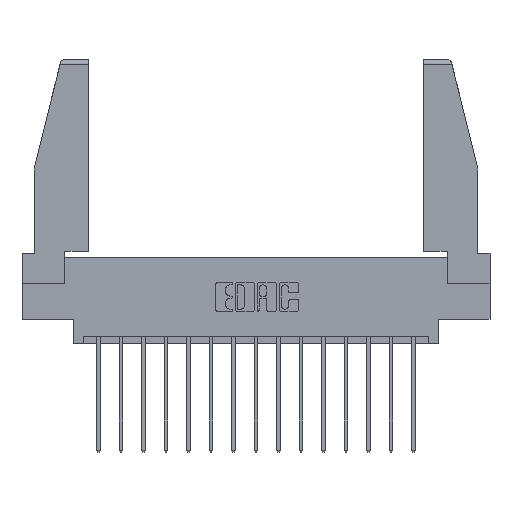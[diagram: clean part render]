
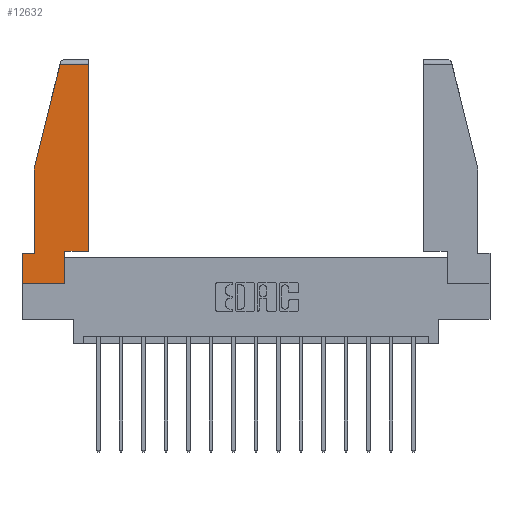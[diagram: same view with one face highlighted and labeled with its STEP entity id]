
A CAD part, top view. The second image highlights one B-rep face of the part: STEP entity #12632.
In plain terms, the highlighted planar face has unit normal (0, 0, 1).
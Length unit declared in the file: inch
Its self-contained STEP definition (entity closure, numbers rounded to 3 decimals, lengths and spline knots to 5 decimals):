
#49 = VERTEX_POINT ( 'NONE', #2338 ) ;
#103 = VERTEX_POINT ( 'NONE', #572 ) ;
#453 = VECTOR ( 'NONE', #15918, 39.37008 ) ;
#572 = CARTESIAN_POINT ( 'NONE',  ( 0.086, 0.8, 0. ) ) ;
#788 = LINE ( 'NONE', #13506, #8327 ) ;
#1800 = DIRECTION ( 'NONE',  ( 0., 1., 0. ) ) ;
#1918 = CARTESIAN_POINT ( 'NONE',  ( 0.297, 0., 0. ) ) ;
#2338 = CARTESIAN_POINT ( 'NONE',  ( 0.2636, 1.52, 0. ) ) ;
#2360 = DIRECTION ( 'NONE',  ( 0., -1., 0. ) ) ;
#2427 = DIRECTION ( 'NONE',  ( 0., 0., 1. ) ) ;
#2500 = CARTESIAN_POINT ( 'NONE',  ( 0.297, 0., 0. ) ) ;
#2665 = EDGE_CURVE ( 'NONE', #16156, #49, #3966, .T. ) ;
#2792 = VECTOR ( 'NONE', #6861, 39.37008 ) ;
#2882 = VERTEX_POINT ( 'NONE', #13273 ) ;
#2923 = CARTESIAN_POINT ( 'NONE',  ( 0.461, 1.52, 0. ) ) ;
#2951 = CARTESIAN_POINT ( 'NONE',  ( 0.271, 1.55, 0. ) ) ;
#3058 = EDGE_CURVE ( 'NONE', #49, #103, #9755, .T. ) ;
#3072 = LINE ( 'NONE', #9177, #17648 ) ;
#3100 = VECTOR ( 'NONE', #1800, 39.37008 ) ;
#3397 = VERTEX_POINT ( 'NONE', #14018 ) ;
#3966 = LINE ( 'NONE', #11786, #8070 ) ;
#4071 = FACE_OUTER_BOUND ( 'NONE', #16138, .T. ) ;
#4286 = ORIENTED_EDGE ( 'NONE', *, *, #14082, .T. ) ;
#4375 = VERTEX_POINT ( 'NONE', #8922 ) ;
#4396 = VECTOR ( 'NONE', #5967, 39.37008 ) ;
#4935 = LINE ( 'NONE', #6620, #14183 ) ;
#5176 = DIRECTION ( 'NONE',  ( 0., -1., 0. ) ) ;
#5409 = EDGE_CURVE ( 'NONE', #5572, #4375, #14403, .T. ) ;
#5572 = VERTEX_POINT ( 'NONE', #11975 ) ;
#5713 = EDGE_CURVE ( 'NONE', #2882, #3397, #10502, .T. ) ;
#5967 = DIRECTION ( 'NONE',  ( -0.239, -0.971, 0. ) ) ;
#6068 = ORIENTED_EDGE ( 'NONE', *, *, #9180, .T. ) ;
#6324 = ORIENTED_EDGE ( 'NONE', *, *, #3058, .T. ) ;
#6438 = ORIENTED_EDGE ( 'NONE', *, *, #15365, .T. ) ;
#6620 = CARTESIAN_POINT ( 'NONE',  ( 0.461, 0.223, 0. ) ) ;
#6753 = ORIENTED_EDGE ( 'NONE', *, *, #2665, .T. ) ;
#6861 = DIRECTION ( 'NONE',  ( -1., 0., 0. ) ) ;
#7098 = VECTOR ( 'NONE', #5176, 39.37008 ) ;
#8070 = VECTOR ( 'NONE', #10594, 39.37008 ) ;
#8327 = VECTOR ( 'NONE', #2360, 39.37008 ) ;
#8391 = LINE ( 'NONE', #12028, #7098 ) ;
#8483 = CARTESIAN_POINT ( 'NONE',  ( 0., 0.21, 0. ) ) ;
#8702 = LINE ( 'NONE', #1918, #3100 ) ;
#8922 = CARTESIAN_POINT ( 'NONE',  ( 0.461, 0.223, 0. ) ) ;
#9068 = DIRECTION ( 'NONE',  ( 1., 0., 0. ) ) ;
#9177 = CARTESIAN_POINT ( 'NONE',  ( 0., 0., 0. ) ) ;
#9180 = EDGE_CURVE ( 'NONE', #103, #2882, #788, .T. ) ;
#9755 = LINE ( 'NONE', #2951, #4396 ) ;
#10502 = LINE ( 'NONE', #8483, #2792 ) ;
#10594 = DIRECTION ( 'NONE',  ( -1., 0., 0. ) ) ;
#10842 = DIRECTION ( 'NONE',  ( 0., 1., 0. ) ) ;
#11786 = CARTESIAN_POINT ( 'NONE',  ( 0., 1.52, 0. ) ) ;
#11975 = CARTESIAN_POINT ( 'NONE',  ( 0.297, 0.223, 0. ) ) ;
#12028 = CARTESIAN_POINT ( 'NONE',  ( 0., 0.21, 0. ) ) ;
#12632 = ADVANCED_FACE ( 'NONE', ( #4071 ), #14561, .T. ) ;
#12910 = ORIENTED_EDGE ( 'NONE', *, *, #13125, .T. ) ;
#13083 = CARTESIAN_POINT ( 'NONE',  ( 0., 0., 0. ) ) ;
#13125 = EDGE_CURVE ( 'NONE', #3397, #17707, #8391, .T. ) ;
#13273 = CARTESIAN_POINT ( 'NONE',  ( 0.086, 0.21, 0. ) ) ;
#13400 = DIRECTION ( 'NONE',  ( 1., 0., 0. ) ) ;
#13506 = CARTESIAN_POINT ( 'NONE',  ( 0.086, 0.8, 0. ) ) ;
#13841 = AXIS2_PLACEMENT_3D ( 'NONE', #17573, #2427, #13400 ) ;
#14018 = CARTESIAN_POINT ( 'NONE',  ( 0., 0.21, 0. ) ) ;
#14082 = EDGE_CURVE ( 'NONE', #15835, #5572, #8702, .T. ) ;
#14183 = VECTOR ( 'NONE', #10842, 39.37008 ) ;
#14403 = LINE ( 'NONE', #17409, #453 ) ;
#14561 = PLANE ( 'NONE',  #13841 ) ;
#15365 = EDGE_CURVE ( 'NONE', #17707, #15835, #3072, .T. ) ;
#15835 = VERTEX_POINT ( 'NONE', #2500 ) ;
#15918 = DIRECTION ( 'NONE',  ( 1., 0., 0. ) ) ;
#16138 = EDGE_LOOP ( 'NONE', ( #17382, #6753, #6324, #6068, #16166, #12910, #6438, #4286, #16220 ) ) ;
#16156 = VERTEX_POINT ( 'NONE', #2923 ) ;
#16166 = ORIENTED_EDGE ( 'NONE', *, *, #5713, .T. ) ;
#16220 = ORIENTED_EDGE ( 'NONE', *, *, #5409, .T. ) ;
#17033 = EDGE_CURVE ( 'NONE', #4375, #16156, #4935, .T. ) ;
#17382 = ORIENTED_EDGE ( 'NONE', *, *, #17033, .T. ) ;
#17409 = CARTESIAN_POINT ( 'NONE',  ( 0.297, 0.223, 0. ) ) ;
#17573 = CARTESIAN_POINT ( 'NONE',  ( 0., 0., 0. ) ) ;
#17648 = VECTOR ( 'NONE', #9068, 39.37008 ) ;
#17707 = VERTEX_POINT ( 'NONE', #13083 ) ;
